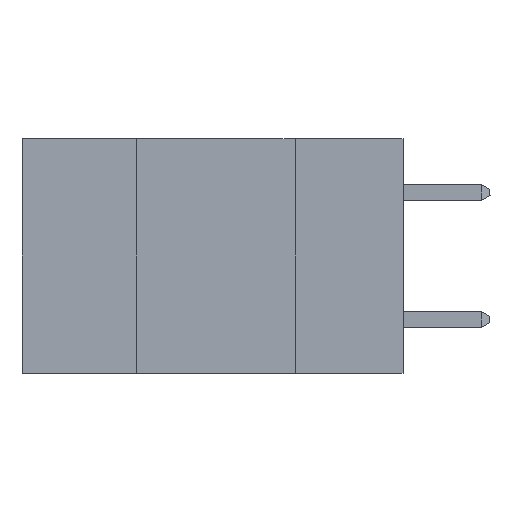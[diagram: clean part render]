
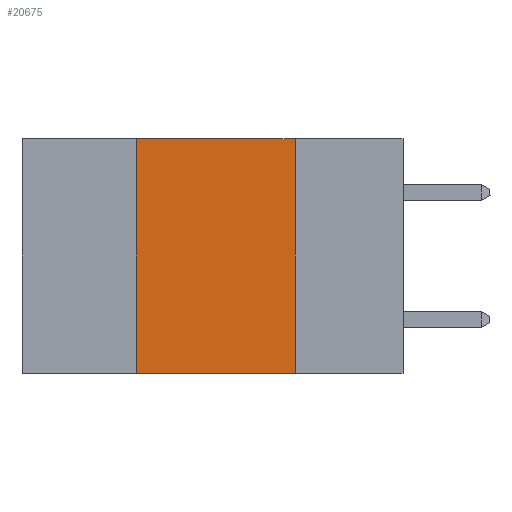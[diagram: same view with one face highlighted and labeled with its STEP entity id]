
A CAD part, left-side view. The second image highlights one B-rep face of the part: STEP entity #20675.
In plain terms, the highlighted planar face has unit normal (-1, 0, 0).
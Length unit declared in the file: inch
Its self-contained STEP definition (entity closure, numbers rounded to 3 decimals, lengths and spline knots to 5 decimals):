
#590 = FACE_OUTER_BOUND ( 'NONE', #6992, .T. ) ;
#761 = EDGE_CURVE ( 'NONE', #32813, #19979, #12464, .T. ) ;
#2991 = CARTESIAN_POINT ( 'NONE',  ( 0., 0.17, -0.37 ) ) ;
#3544 = AXIS2_PLACEMENT_3D ( 'NONE', #30581, #12608, #10115 ) ;
#4698 = DIRECTION ( 'NONE',  ( 0., 0., 1. ) ) ;
#5326 = VERTEX_POINT ( 'NONE', #18944 ) ;
#6992 = EDGE_LOOP ( 'NONE', ( #16776, #19244, #10987, #8952 ) ) ;
#7543 = LINE ( 'NONE', #27844, #27728 ) ;
#8952 = ORIENTED_EDGE ( 'NONE', *, *, #761, .T. ) ;
#9184 = CARTESIAN_POINT ( 'NONE',  ( 0., 0.6, -0.37 ) ) ;
#10115 = DIRECTION ( 'NONE',  ( 0., 0., -1. ) ) ;
#10453 = CARTESIAN_POINT ( 'NONE',  ( 0., 0.42, 0. ) ) ;
#10764 = PLANE ( 'NONE',  #3544 ) ;
#10987 = ORIENTED_EDGE ( 'NONE', *, *, #27529, .F. ) ;
#11433 = LINE ( 'NONE', #21898, #14227 ) ;
#12464 = LINE ( 'NONE', #9184, #19921 ) ;
#12608 = DIRECTION ( 'NONE',  ( 1., 0., 0. ) ) ;
#12703 = CARTESIAN_POINT ( 'NONE',  ( 0., 0.42, -0.37 ) ) ;
#12774 = LINE ( 'NONE', #23082, #13139 ) ;
#13139 = VECTOR ( 'NONE', #28246, 39.37008 ) ;
#14227 = VECTOR ( 'NONE', #32077, 39.37008 ) ;
#16480 = DIRECTION ( 'NONE',  ( 0., -1., 0. ) ) ;
#16776 = ORIENTED_EDGE ( 'NONE', *, *, #20647, .F. ) ;
#18944 = CARTESIAN_POINT ( 'NONE',  ( 0., 0.17, 0. ) ) ;
#19244 = ORIENTED_EDGE ( 'NONE', *, *, #21269, .F. ) ;
#19921 = VECTOR ( 'NONE', #16480, 39.37008 ) ;
#19979 = VERTEX_POINT ( 'NONE', #2991 ) ;
#20647 = EDGE_CURVE ( 'NONE', #5326, #19979, #12774, .T. ) ;
#20675 = ADVANCED_FACE ( 'NONE', ( #590 ), #10764, .F. ) ;
#21269 = EDGE_CURVE ( 'NONE', #28587, #5326, #11433, .T. ) ;
#21898 = CARTESIAN_POINT ( 'NONE',  ( 0., 0.6, 0. ) ) ;
#23082 = CARTESIAN_POINT ( 'NONE',  ( 0., 0.17, 0. ) ) ;
#27529 = EDGE_CURVE ( 'NONE', #32813, #28587, #7543, .T. ) ;
#27728 = VECTOR ( 'NONE', #4698, 39.37008 ) ;
#27844 = CARTESIAN_POINT ( 'NONE',  ( 0., 0.42, 0. ) ) ;
#28246 = DIRECTION ( 'NONE',  ( 0., 0., -1. ) ) ;
#28587 = VERTEX_POINT ( 'NONE', #10453 ) ;
#30581 = CARTESIAN_POINT ( 'NONE',  ( 0., 0.6, 0. ) ) ;
#32077 = DIRECTION ( 'NONE',  ( 0., -1., 0. ) ) ;
#32813 = VERTEX_POINT ( 'NONE', #12703 ) ;
